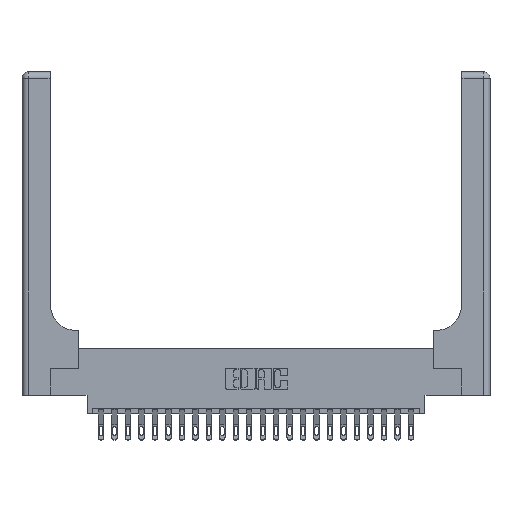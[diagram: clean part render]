
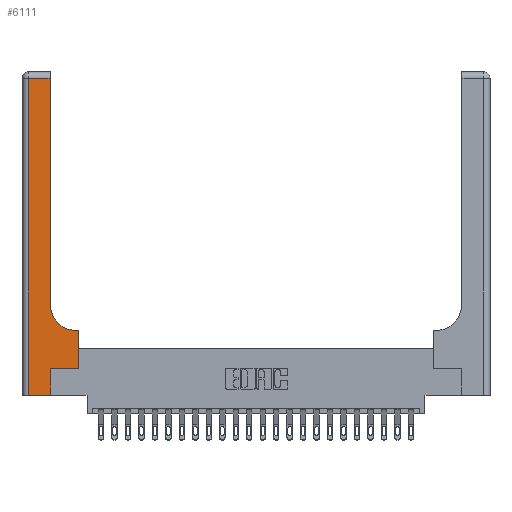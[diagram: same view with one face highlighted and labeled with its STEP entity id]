
A CAD part, top view. The second image highlights one B-rep face of the part: STEP entity #6111.
In plain terms, the highlighted planar face has unit normal (0, 0, 1).
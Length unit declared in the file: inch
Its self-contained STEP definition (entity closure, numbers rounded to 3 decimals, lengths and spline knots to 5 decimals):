
#355 = VERTEX_POINT ( 'NONE', #2155 ) ;
#489 = EDGE_LOOP ( 'NONE', ( #1425, #6252, #4219, #13793, #12165, #4519, #21719, #2678, #2747 ) ) ;
#1425 = ORIENTED_EDGE ( 'NONE', *, *, #2323, .T. ) ;
#1615 = LINE ( 'NONE', #4061, #20588 ) ;
#2155 = CARTESIAN_POINT ( 'NONE',  ( 0.06, 0., 0.37 ) ) ;
#2323 = EDGE_CURVE ( 'NONE', #19940, #11969, #5012, .T. ) ;
#2678 = ORIENTED_EDGE ( 'NONE', *, *, #21401, .T. ) ;
#2747 = ORIENTED_EDGE ( 'NONE', *, *, #22024, .T. ) ;
#2876 = CARTESIAN_POINT ( 'NONE',  ( 0.26, 2.94, 0.37 ) ) ;
#2916 = PLANE ( 'NONE',  #14255 ) ;
#3091 = CARTESIAN_POINT ( 'NONE',  ( 0.528, 0.25, 0.37 ) ) ;
#4061 = CARTESIAN_POINT ( 'NONE',  ( 0.528, 0.25, 0.37 ) ) ;
#4219 = ORIENTED_EDGE ( 'NONE', *, *, #20813, .T. ) ;
#4519 = ORIENTED_EDGE ( 'NONE', *, *, #6210, .T. ) ;
#4757 = DIRECTION ( 'NONE',  ( -1., 0., 0. ) ) ;
#5012 = LINE ( 'NONE', #8826, #5603 ) ;
#5202 = VECTOR ( 'NONE', #9063, 39.37008 ) ;
#5289 = VERTEX_POINT ( 'NONE', #18669 ) ;
#5522 = CARTESIAN_POINT ( 'NONE',  ( 0.265, 0., 0.37 ) ) ;
#5603 = VECTOR ( 'NONE', #10681, 39.37008 ) ;
#6111 = ADVANCED_FACE ( 'NONE', ( #6931 ), #2916, .F. ) ;
#6210 = EDGE_CURVE ( 'NONE', #15245, #9791, #11713, .T. ) ;
#6252 = ORIENTED_EDGE ( 'NONE', *, *, #19571, .T. ) ;
#6497 = EDGE_CURVE ( 'NONE', #9791, #14556, #1615, .T. ) ;
#6875 = DIRECTION ( 'NONE',  ( 0., -1., 0. ) ) ;
#6931 = FACE_OUTER_BOUND ( 'NONE', #489, .T. ) ;
#6962 = VECTOR ( 'NONE', #16531, 39.37008 ) ;
#7823 = CARTESIAN_POINT ( 'NONE',  ( 0.265, 0.25, 0.37 ) ) ;
#8411 = DIRECTION ( 'NONE',  ( 0., 0., -1. ) ) ;
#8826 = CARTESIAN_POINT ( 'NONE',  ( 0.26, 3., 0.37 ) ) ;
#9063 = DIRECTION ( 'NONE',  ( 1., 0., 0. ) ) ;
#9425 = EDGE_CURVE ( 'NONE', #5289, #15245, #16147, .T. ) ;
#9791 = VERTEX_POINT ( 'NONE', #3091 ) ;
#10209 = VECTOR ( 'NONE', #17594, 39.37008 ) ;
#10236 = CARTESIAN_POINT ( 'NONE',  ( 0.26, 0.6, 0.37 ) ) ;
#10261 = CARTESIAN_POINT ( 'NONE',  ( 0.51, 0.85, 0.37 ) ) ;
#10290 = CARTESIAN_POINT ( 'NONE',  ( 0.06, 2.94, 0.37 ) ) ;
#10681 = DIRECTION ( 'NONE',  ( 0., 1., 0. ) ) ;
#11713 = LINE ( 'NONE', #19438, #16011 ) ;
#11969 = VERTEX_POINT ( 'NONE', #2876 ) ;
#12087 = CARTESIAN_POINT ( 'NONE',  ( 0., 3., 0.37 ) ) ;
#12093 = DIRECTION ( 'NONE',  ( 1., 0., 0. ) ) ;
#12165 = ORIENTED_EDGE ( 'NONE', *, *, #9425, .T. ) ;
#12742 = CARTESIAN_POINT ( 'NONE',  ( 0., 0., 0.37 ) ) ;
#12748 = CIRCLE ( 'NONE', #23095, 0.25 ) ;
#13793 = ORIENTED_EDGE ( 'NONE', *, *, #23366, .T. ) ;
#14122 = VERTEX_POINT ( 'NONE', #10290 ) ;
#14250 = DIRECTION ( 'NONE',  ( -1., 0., 0. ) ) ;
#14255 = AXIS2_PLACEMENT_3D ( 'NONE', #12087, #8411, #4757 ) ;
#14556 = VERTEX_POINT ( 'NONE', #22354 ) ;
#15089 = LINE ( 'NONE', #10236, #10209 ) ;
#15102 = DIRECTION ( 'NONE',  ( 0., 1., 0. ) ) ;
#15245 = VERTEX_POINT ( 'NONE', #7823 ) ;
#15264 = CARTESIAN_POINT ( 'NONE',  ( 0.26, 0.85, 0.37 ) ) ;
#15919 = CARTESIAN_POINT ( 'NONE',  ( 0.51, 0.6, 0.37 ) ) ;
#16011 = VECTOR ( 'NONE', #17659, 39.37008 ) ;
#16147 = LINE ( 'NONE', #5522, #6962 ) ;
#16531 = DIRECTION ( 'NONE',  ( 0., 1., 0. ) ) ;
#17389 = VECTOR ( 'NONE', #6875, 39.37008 ) ;
#17594 = DIRECTION ( 'NONE',  ( -1., 0., 0. ) ) ;
#17659 = DIRECTION ( 'NONE',  ( 1., 0., 0. ) ) ;
#17742 = LINE ( 'NONE', #23336, #22040 ) ;
#18669 = CARTESIAN_POINT ( 'NONE',  ( 0.265, 0., 0.37 ) ) ;
#19438 = CARTESIAN_POINT ( 'NONE',  ( 0.265, 0.25, 0.37 ) ) ;
#19571 = EDGE_CURVE ( 'NONE', #11969, #14122, #17742, .T. ) ;
#19859 = LINE ( 'NONE', #12742, #5202 ) ;
#19940 = VERTEX_POINT ( 'NONE', #15264 ) ;
#20588 = VECTOR ( 'NONE', #15102, 39.37008 ) ;
#20813 = EDGE_CURVE ( 'NONE', #14122, #355, #23389, .T. ) ;
#21401 = EDGE_CURVE ( 'NONE', #14556, #21453, #15089, .T. ) ;
#21453 = VERTEX_POINT ( 'NONE', #15919 ) ;
#21543 = CARTESIAN_POINT ( 'NONE',  ( 0.06, 3., 0.37 ) ) ;
#21719 = ORIENTED_EDGE ( 'NONE', *, *, #6497, .T. ) ;
#22024 = EDGE_CURVE ( 'NONE', #21453, #19940, #12748, .T. ) ;
#22040 = VECTOR ( 'NONE', #14250, 39.37008 ) ;
#22354 = CARTESIAN_POINT ( 'NONE',  ( 0.528, 0.6, 0.37 ) ) ;
#23049 = DIRECTION ( 'NONE',  ( 0., 0., -1. ) ) ;
#23095 = AXIS2_PLACEMENT_3D ( 'NONE', #10261, #23049, #12093 ) ;
#23336 = CARTESIAN_POINT ( 'NONE',  ( 0., 2.94, 0.37 ) ) ;
#23366 = EDGE_CURVE ( 'NONE', #355, #5289, #19859, .T. ) ;
#23389 = LINE ( 'NONE', #21543, #17389 ) ;
